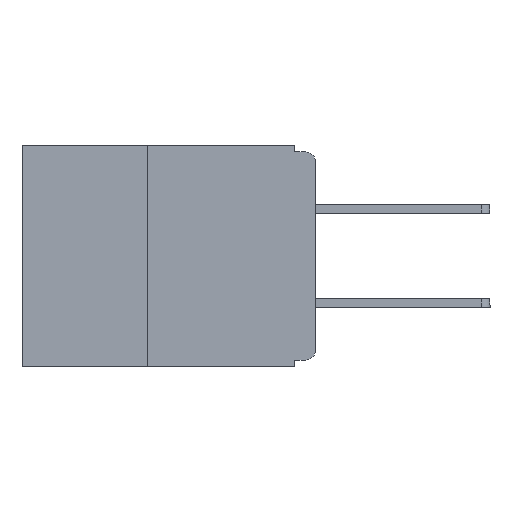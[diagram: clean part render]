
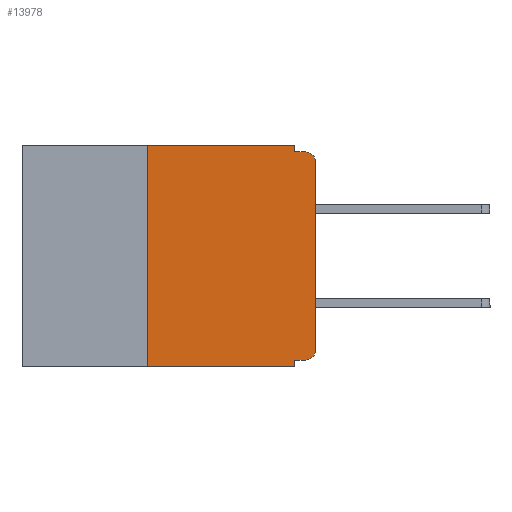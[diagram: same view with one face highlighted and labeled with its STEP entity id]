
A CAD part, left-side view. The second image highlights one B-rep face of the part: STEP entity #13978.
In plain terms, the highlighted planar face has unit normal (-1, 0, 0).
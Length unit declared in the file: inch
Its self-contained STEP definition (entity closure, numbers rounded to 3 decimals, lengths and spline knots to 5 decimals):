
#200 = DIRECTION ( 'NONE',  ( 0., 0., -1. ) ) ;
#611 = VERTEX_POINT ( 'NONE', #22471 ) ;
#1734 = ORIENTED_EDGE ( 'NONE', *, *, #4400, .T. ) ;
#1799 = DIRECTION ( 'NONE',  ( 0., 0., -1. ) ) ;
#1869 = VERTEX_POINT ( 'NONE', #17471 ) ;
#2432 = LINE ( 'NONE', #14604, #6896 ) ;
#2607 = CARTESIAN_POINT ( 'NONE',  ( 0., 0., 0. ) ) ;
#2882 = LINE ( 'NONE', #18714, #21463 ) ;
#3131 = EDGE_CURVE ( 'NONE', #611, #9164, #3269, .T. ) ;
#3269 = LINE ( 'NONE', #9430, #12705 ) ;
#3331 = DIRECTION ( 'NONE',  ( 0., 1., 0. ) ) ;
#3535 = CARTESIAN_POINT ( 'NONE',  ( 0., 0.015, -0.32 ) ) ;
#4264 = VECTOR ( 'NONE', #15812, 39.37008 ) ;
#4269 = EDGE_LOOP ( 'NONE', ( #5681, #19688, #8732, #4920, #6831, #16668, #1734, #11655, #18647, #9076 ) ) ;
#4400 = EDGE_CURVE ( 'NONE', #13669, #9164, #23562, .T. ) ;
#4637 = DIRECTION ( 'NONE',  ( 0., -1., 0. ) ) ;
#4920 = ORIENTED_EDGE ( 'NONE', *, *, #9441, .F. ) ;
#4973 = VERTEX_POINT ( 'NONE', #6339 ) ;
#5058 = EDGE_CURVE ( 'NONE', #1869, #19485, #9286, .T. ) ;
#5672 = EDGE_CURVE ( 'NONE', #13669, #4973, #16789, .T. ) ;
#5681 = ORIENTED_EDGE ( 'NONE', *, *, #5058, .T. ) ;
#6339 = CARTESIAN_POINT ( 'NONE',  ( 0., 0.25, 0. ) ) ;
#6773 = VERTEX_POINT ( 'NONE', #22729 ) ;
#6789 = EDGE_CURVE ( 'NONE', #9886, #1869, #16769, .T. ) ;
#6831 = ORIENTED_EDGE ( 'NONE', *, *, #9979, .F. ) ;
#6896 = VECTOR ( 'NONE', #3331, 39.37008 ) ;
#6909 = VECTOR ( 'NONE', #15708, 39.37008 ) ;
#6928 = CARTESIAN_POINT ( 'NONE',  ( 0., 0.25, -0.33 ) ) ;
#7883 = CARTESIAN_POINT ( 'NONE',  ( 0., 0.031, 0. ) ) ;
#8151 = CARTESIAN_POINT ( 'NONE',  ( 0., 0.015, -0.305 ) ) ;
#8506 = DIRECTION ( 'NONE',  ( 0., 0., -1. ) ) ;
#8732 = ORIENTED_EDGE ( 'NONE', *, *, #21624, .F. ) ;
#9076 = ORIENTED_EDGE ( 'NONE', *, *, #6789, .T. ) ;
#9164 = VERTEX_POINT ( 'NONE', #23515 ) ;
#9286 = LINE ( 'NONE', #2607, #4264 ) ;
#9299 = EDGE_CURVE ( 'NONE', #19485, #11383, #9415, .T. ) ;
#9415 = CIRCLE ( 'NONE', #18071, 0.015 ) ;
#9430 = CARTESIAN_POINT ( 'NONE',  ( 0., 0.031, -0.33 ) ) ;
#9441 = EDGE_CURVE ( 'NONE', #18454, #6773, #10291, .T. ) ;
#9545 = FACE_OUTER_BOUND ( 'NONE', #4269, .T. ) ;
#9698 = CARTESIAN_POINT ( 'NONE',  ( 0., 0.437, 0. ) ) ;
#9886 = VERTEX_POINT ( 'NONE', #3535 ) ;
#9979 = EDGE_CURVE ( 'NONE', #4973, #18454, #2882, .T. ) ;
#10033 = DIRECTION ( 'NONE',  ( 0., 0., -1. ) ) ;
#10291 = LINE ( 'NONE', #7883, #19555 ) ;
#11383 = VERTEX_POINT ( 'NONE', #19643 ) ;
#11589 = DIRECTION ( 'NONE',  ( 1., 0., 0. ) ) ;
#11655 = ORIENTED_EDGE ( 'NONE', *, *, #3131, .F. ) ;
#12705 = VECTOR ( 'NONE', #8506, 39.37008 ) ;
#13001 = CARTESIAN_POINT ( 'NONE',  ( 0., 0.031, 0. ) ) ;
#13139 = DIRECTION ( 'NONE',  ( -1., 0., 0. ) ) ;
#13669 = VERTEX_POINT ( 'NONE', #6928 ) ;
#13978 = ADVANCED_FACE ( 'NONE', ( #9545 ), #20731, .F. ) ;
#14058 = VECTOR ( 'NONE', #4637, 39.37008 ) ;
#14352 = EDGE_CURVE ( 'NONE', #9886, #611, #2432, .T. ) ;
#14604 = CARTESIAN_POINT ( 'NONE',  ( 0., 0., -0.32 ) ) ;
#15708 = DIRECTION ( 'NONE',  ( 0., 0., 1. ) ) ;
#15812 = DIRECTION ( 'NONE',  ( 0., 0., 1. ) ) ;
#15840 = CARTESIAN_POINT ( 'NONE',  ( 0., 0.437, -0.33 ) ) ;
#16668 = ORIENTED_EDGE ( 'NONE', *, *, #5672, .F. ) ;
#16688 = CARTESIAN_POINT ( 'NONE',  ( 0., 0., -0.025 ) ) ;
#16769 = CIRCLE ( 'NONE', #20923, 0.015 ) ;
#16789 = LINE ( 'NONE', #21183, #6909 ) ;
#16890 = AXIS2_PLACEMENT_3D ( 'NONE', #9698, #11589, #200 ) ;
#17471 = CARTESIAN_POINT ( 'NONE',  ( 0., 0., -0.305 ) ) ;
#17805 = DIRECTION ( 'NONE',  ( 0., -1., 0. ) ) ;
#18071 = AXIS2_PLACEMENT_3D ( 'NONE', #23904, #13139, #1799 ) ;
#18454 = VERTEX_POINT ( 'NONE', #13001 ) ;
#18647 = ORIENTED_EDGE ( 'NONE', *, *, #14352, .F. ) ;
#18714 = CARTESIAN_POINT ( 'NONE',  ( 0., 0.437, 0. ) ) ;
#19485 = VERTEX_POINT ( 'NONE', #16688 ) ;
#19555 = VECTOR ( 'NONE', #22547, 39.37008 ) ;
#19643 = CARTESIAN_POINT ( 'NONE',  ( 0., 0.015, -0.01 ) ) ;
#19688 = ORIENTED_EDGE ( 'NONE', *, *, #9299, .T. ) ;
#19912 = LINE ( 'NONE', #23105, #24011 ) ;
#20530 = DIRECTION ( 'NONE',  ( 0., -1., 0. ) ) ;
#20731 = PLANE ( 'NONE',  #16890 ) ;
#20923 = AXIS2_PLACEMENT_3D ( 'NONE', #8151, #21049, #10033 ) ;
#21049 = DIRECTION ( 'NONE',  ( -1., 0., 0. ) ) ;
#21183 = CARTESIAN_POINT ( 'NONE',  ( 0., 0.25, -0.33 ) ) ;
#21463 = VECTOR ( 'NONE', #20530, 39.37008 ) ;
#21624 = EDGE_CURVE ( 'NONE', #6773, #11383, #19912, .T. ) ;
#22471 = CARTESIAN_POINT ( 'NONE',  ( 0., 0.031, -0.32 ) ) ;
#22547 = DIRECTION ( 'NONE',  ( 0., 0., -1. ) ) ;
#22729 = CARTESIAN_POINT ( 'NONE',  ( 0., 0.031, -0.01 ) ) ;
#23105 = CARTESIAN_POINT ( 'NONE',  ( 0., 0., -0.01 ) ) ;
#23515 = CARTESIAN_POINT ( 'NONE',  ( 0., 0.031, -0.33 ) ) ;
#23562 = LINE ( 'NONE', #15840, #14058 ) ;
#23904 = CARTESIAN_POINT ( 'NONE',  ( 0., 0.015, -0.025 ) ) ;
#24011 = VECTOR ( 'NONE', #17805, 39.37008 ) ;
